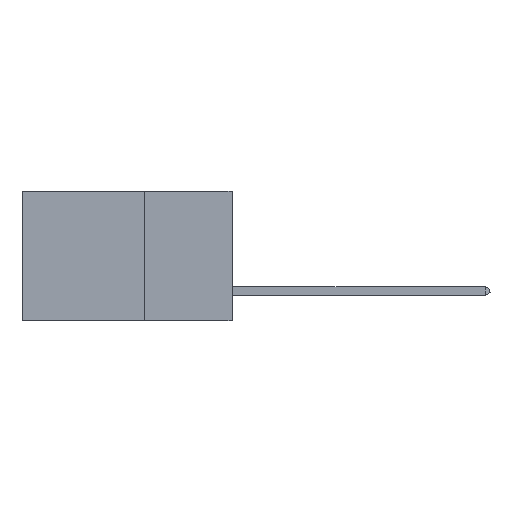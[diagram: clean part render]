
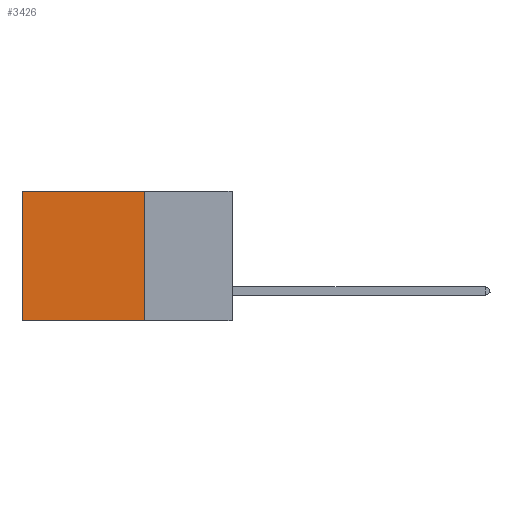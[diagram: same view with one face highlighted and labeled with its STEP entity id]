
A CAD part, left-side view. The second image highlights one B-rep face of the part: STEP entity #3426.
In plain terms, the highlighted planar face has unit normal (-1, 0, 0).
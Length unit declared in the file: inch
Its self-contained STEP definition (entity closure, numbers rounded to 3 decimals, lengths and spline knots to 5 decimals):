
#95 = EDGE_CURVE ( 'NONE', #23311, #8143, #1721, .T. ) ;
#314 = VECTOR ( 'NONE', #2501, 39.37008 ) ;
#386 = DIRECTION ( 'NONE',  ( 0., 1., 0. ) ) ;
#761 = VERTEX_POINT ( 'NONE', #17176 ) ;
#1657 = DIRECTION ( 'NONE',  ( 0., 1., 0. ) ) ;
#1721 = LINE ( 'NONE', #2121, #8217 ) ;
#2121 = CARTESIAN_POINT ( 'NONE',  ( 0.2875, 0.25, 0. ) ) ;
#2501 = DIRECTION ( 'NONE',  ( 0., 0., -1. ) ) ;
#3426 = ADVANCED_FACE ( 'NONE', ( #13172 ), #14715, .F. ) ;
#3673 = CARTESIAN_POINT ( 'NONE',  ( 0.2875, 0.25, 0. ) ) ;
#3830 = DIRECTION ( 'NONE',  ( 0., 0., -1. ) ) ;
#4666 = VERTEX_POINT ( 'NONE', #17765 ) ;
#5640 = CARTESIAN_POINT ( 'NONE',  ( 0.2875, 0.25, 0. ) ) ;
#5744 = LINE ( 'NONE', #9532, #6292 ) ;
#6292 = VECTOR ( 'NONE', #386, 39.37008 ) ;
#8050 = ORIENTED_EDGE ( 'NONE', *, *, #16055, .F. ) ;
#8143 = VERTEX_POINT ( 'NONE', #14650 ) ;
#8217 = VECTOR ( 'NONE', #1657, 39.37008 ) ;
#9532 = CARTESIAN_POINT ( 'NONE',  ( 0.2875, 0.25, -0.37 ) ) ;
#9987 = LINE ( 'NONE', #11456, #314 ) ;
#11456 = CARTESIAN_POINT ( 'NONE',  ( 0.2875, 0.6, 0. ) ) ;
#12735 = VECTOR ( 'NONE', #3830, 39.37008 ) ;
#13051 = EDGE_CURVE ( 'NONE', #8143, #761, #9987, .T. ) ;
#13172 = FACE_OUTER_BOUND ( 'NONE', #19246, .T. ) ;
#14650 = CARTESIAN_POINT ( 'NONE',  ( 0.2875, 0.6, 0. ) ) ;
#14715 = PLANE ( 'NONE',  #21015 ) ;
#14756 = ORIENTED_EDGE ( 'NONE', *, *, #95, .T. ) ;
#14937 = DIRECTION ( 'NONE',  ( 0., 0., -1. ) ) ;
#14989 = LINE ( 'NONE', #19991, #12735 ) ;
#15205 = ORIENTED_EDGE ( 'NONE', *, *, #18047, .F. ) ;
#16055 = EDGE_CURVE ( 'NONE', #4666, #761, #5744, .T. ) ;
#17176 = CARTESIAN_POINT ( 'NONE',  ( 0.2875, 0.6, -0.37 ) ) ;
#17765 = CARTESIAN_POINT ( 'NONE',  ( 0.2875, 0.25, -0.37 ) ) ;
#18047 = EDGE_CURVE ( 'NONE', #23311, #4666, #14989, .T. ) ;
#18261 = DIRECTION ( 'NONE',  ( 1., 0., 0. ) ) ;
#19246 = EDGE_LOOP ( 'NONE', ( #20877, #8050, #15205, #14756 ) ) ;
#19991 = CARTESIAN_POINT ( 'NONE',  ( 0.2875, 0.25, 0. ) ) ;
#20877 = ORIENTED_EDGE ( 'NONE', *, *, #13051, .T. ) ;
#21015 = AXIS2_PLACEMENT_3D ( 'NONE', #5640, #18261, #14937 ) ;
#23311 = VERTEX_POINT ( 'NONE', #3673 ) ;
